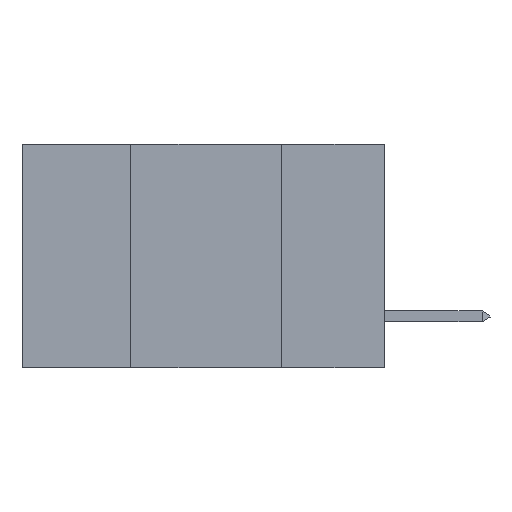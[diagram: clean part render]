
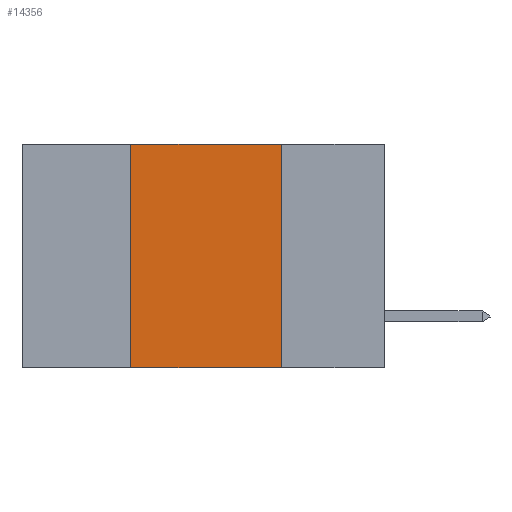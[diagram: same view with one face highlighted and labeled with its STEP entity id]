
A CAD part, left-side view. The second image highlights one B-rep face of the part: STEP entity #14356.
In plain terms, the highlighted planar face has unit normal (-1, 0, 0).
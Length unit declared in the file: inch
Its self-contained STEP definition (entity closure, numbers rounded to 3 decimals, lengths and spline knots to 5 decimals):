
#1226 = EDGE_CURVE ( 'NONE', #8561, #7398, #18532, .T. ) ;
#1309 = ORIENTED_EDGE ( 'NONE', *, *, #16541, .F. ) ;
#1381 = VECTOR ( 'NONE', #3109, 39.37008 ) ;
#2085 = VECTOR ( 'NONE', #10869, 39.37008 ) ;
#2308 = ORIENTED_EDGE ( 'NONE', *, *, #1226, .F. ) ;
#3062 = PLANE ( 'NONE',  #12365 ) ;
#3109 = DIRECTION ( 'NONE',  ( 0., 0., -1. ) ) ;
#3194 = DIRECTION ( 'NONE',  ( 1., 0., 0. ) ) ;
#3570 = CARTESIAN_POINT ( 'NONE',  ( 0., 0.6, 0. ) ) ;
#4741 = EDGE_CURVE ( 'NONE', #6334, #7398, #12757, .T. ) ;
#6334 = VERTEX_POINT ( 'NONE', #12842 ) ;
#6463 = CARTESIAN_POINT ( 'NONE',  ( 0., 0.42, 0. ) ) ;
#6645 = ORIENTED_EDGE ( 'NONE', *, *, #11394, .F. ) ;
#6770 = CARTESIAN_POINT ( 'NONE',  ( 0., 0.17, 0. ) ) ;
#7258 = CARTESIAN_POINT ( 'NONE',  ( 0., 0.6, -0.37 ) ) ;
#7398 = VERTEX_POINT ( 'NONE', #15579 ) ;
#8561 = VERTEX_POINT ( 'NONE', #17983 ) ;
#9286 = DIRECTION ( 'NONE',  ( 0., 0., -1. ) ) ;
#9435 = LINE ( 'NONE', #3570, #16271 ) ;
#10079 = VERTEX_POINT ( 'NONE', #17413 ) ;
#10869 = DIRECTION ( 'NONE',  ( 0., 0., 1. ) ) ;
#11129 = FACE_OUTER_BOUND ( 'NONE', #11957, .T. ) ;
#11394 = EDGE_CURVE ( 'NONE', #6334, #10079, #19485, .T. ) ;
#11957 = EDGE_LOOP ( 'NONE', ( #2308, #1309, #6645, #12083 ) ) ;
#12083 = ORIENTED_EDGE ( 'NONE', *, *, #4741, .T. ) ;
#12365 = AXIS2_PLACEMENT_3D ( 'NONE', #13545, #3194, #9286 ) ;
#12757 = LINE ( 'NONE', #7258, #18642 ) ;
#12842 = CARTESIAN_POINT ( 'NONE',  ( 0., 0.42, -0.37 ) ) ;
#13545 = CARTESIAN_POINT ( 'NONE',  ( 0., 0.6, 0. ) ) ;
#14356 = ADVANCED_FACE ( 'NONE', ( #11129 ), #3062, .F. ) ;
#15579 = CARTESIAN_POINT ( 'NONE',  ( 0., 0.17, -0.37 ) ) ;
#16271 = VECTOR ( 'NONE', #18557, 39.37008 ) ;
#16541 = EDGE_CURVE ( 'NONE', #10079, #8561, #9435, .T. ) ;
#17413 = CARTESIAN_POINT ( 'NONE',  ( 0., 0.42, 0. ) ) ;
#17869 = DIRECTION ( 'NONE',  ( 0., -1., 0. ) ) ;
#17983 = CARTESIAN_POINT ( 'NONE',  ( 0., 0.17, 0. ) ) ;
#18532 = LINE ( 'NONE', #6770, #1381 ) ;
#18557 = DIRECTION ( 'NONE',  ( 0., -1., 0. ) ) ;
#18642 = VECTOR ( 'NONE', #17869, 39.37008 ) ;
#19485 = LINE ( 'NONE', #6463, #2085 ) ;
